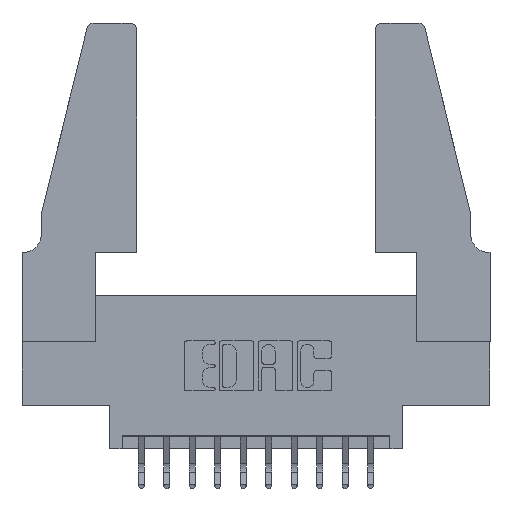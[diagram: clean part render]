
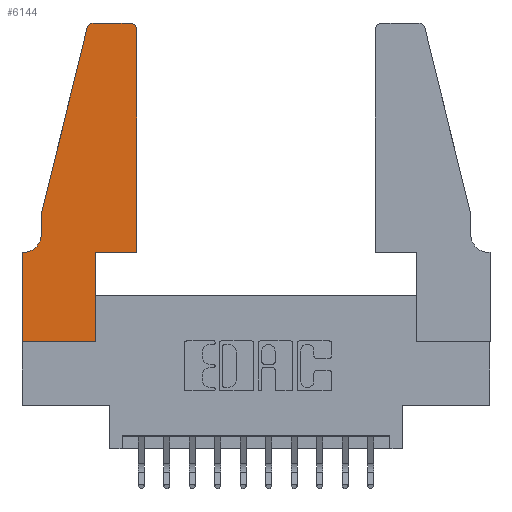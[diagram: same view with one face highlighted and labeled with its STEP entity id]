
A CAD part, top view. The second image highlights one B-rep face of the part: STEP entity #6144.
In plain terms, the highlighted planar face has unit normal (0, 0, 1).
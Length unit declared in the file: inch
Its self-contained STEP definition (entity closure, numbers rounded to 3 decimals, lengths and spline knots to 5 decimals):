
#168 = LINE ( 'NONE', #5309, #11917 ) ;
#169 = CARTESIAN_POINT ( 'NONE',  ( 0.0055, 0.35, 0.37 ) ) ;
#407 = EDGE_CURVE ( 'NONE', #7025, #11559, #3150, .T. ) ;
#533 = DIRECTION ( 'NONE',  ( 1., 0., 0. ) ) ;
#986 = CARTESIAN_POINT ( 'NONE',  ( 0.4505, 1.22, 0.37 ) ) ;
#995 = EDGE_LOOP ( 'NONE', ( #4113, #4151, #4274, #4350, #4409, #4457, #4525, #4723, #4753, #4770, #4849, #4875 ) ) ;
#1064 = DIRECTION ( 'NONE',  ( 0., 0., 1. ) ) ;
#1070 = CARTESIAN_POINT ( 'NONE',  ( 0.0755, 0.42, 0.37 ) ) ;
#1139 = CIRCLE ( 'NONE', #1979, 0.07 ) ;
#1775 = EDGE_CURVE ( 'NONE', #12695, #11120, #4900, .T. ) ;
#1860 = VECTOR ( 'NONE', #6840, 39.37008 ) ;
#1902 = CARTESIAN_POINT ( 'NONE',  ( 0.4205, 1.25, 0.37 ) ) ;
#1979 = AXIS2_PLACEMENT_3D ( 'NONE', #4079, #11868, #5188 ) ;
#2409 = EDGE_CURVE ( 'NONE', #10129, #10634, #13454, .T. ) ;
#2647 = EDGE_CURVE ( 'NONE', #4842, #14044, #4719, .T. ) ;
#3150 = LINE ( 'NONE', #5329, #8751 ) ;
#3224 = DIRECTION ( 'NONE',  ( 0., -1., 0. ) ) ;
#3579 = VERTEX_POINT ( 'NONE', #986 ) ;
#3812 = EDGE_CURVE ( 'NONE', #10634, #3579, #11188, .T. ) ;
#4055 = CARTESIAN_POINT ( 'NONE',  ( 0., 0.35, 0.37 ) ) ;
#4079 = CARTESIAN_POINT ( 'NONE',  ( 0.0055, 0.42, 0.37 ) ) ;
#4113 = ORIENTED_EDGE ( 'NONE', *, *, #12230, .T. ) ;
#4151 = ORIENTED_EDGE ( 'NONE', *, *, #2647, .T. ) ;
#4274 = ORIENTED_EDGE ( 'NONE', *, *, #13954, .T. ) ;
#4350 = ORIENTED_EDGE ( 'NONE', *, *, #1775, .T. ) ;
#4362 = VECTOR ( 'NONE', #4986, 39.37008 ) ;
#4409 = ORIENTED_EDGE ( 'NONE', *, *, #9693, .T. ) ;
#4457 = ORIENTED_EDGE ( 'NONE', *, *, #407, .T. ) ;
#4491 = VERTEX_POINT ( 'NONE', #4540 ) ;
#4525 = ORIENTED_EDGE ( 'NONE', *, *, #8069, .T. ) ;
#4540 = CARTESIAN_POINT ( 'NONE',  ( 0.2865, 0., 0.37 ) ) ;
#4719 = CIRCLE ( 'NONE', #12074, 0.03 ) ;
#4723 = ORIENTED_EDGE ( 'NONE', *, *, #12781, .T. ) ;
#4753 = ORIENTED_EDGE ( 'NONE', *, *, #14152, .T. ) ;
#4770 = ORIENTED_EDGE ( 'NONE', *, *, #2409, .T. ) ;
#4842 = VERTEX_POINT ( 'NONE', #10704 ) ;
#4849 = ORIENTED_EDGE ( 'NONE', *, *, #3812, .T. ) ;
#4875 = ORIENTED_EDGE ( 'NONE', *, *, #8145, .T. ) ;
#4900 = LINE ( 'NONE', #14087, #13107 ) ;
#4986 = DIRECTION ( 'NONE',  ( -0.239, -0.971, 0. ) ) ;
#5111 = PLANE ( 'NONE',  #6450 ) ;
#5149 = CARTESIAN_POINT ( 'NONE',  ( 0., 0., 0.37 ) ) ;
#5188 = DIRECTION ( 'NONE',  ( -1., 0., 0. ) ) ;
#5261 = LINE ( 'NONE', #5149, #10844 ) ;
#5309 = CARTESIAN_POINT ( 'NONE',  ( 0.2605, 1.25, 0.37 ) ) ;
#5329 = CARTESIAN_POINT ( 'NONE',  ( 0.0755, 0.35, 0.37 ) ) ;
#5587 = VERTEX_POINT ( 'NONE', #1902 ) ;
#5948 = CARTESIAN_POINT ( 'NONE',  ( 0.2865, 0.35, 0.37 ) ) ;
#6144 = ADVANCED_FACE ( 'NONE', ( #10615 ), #5111, .T. ) ;
#6252 = DIRECTION ( 'NONE',  ( 1., 0., 0. ) ) ;
#6427 = DIRECTION ( 'NONE',  ( -1., 0., 0. ) ) ;
#6450 = AXIS2_PLACEMENT_3D ( 'NONE', #4055, #7343, #533 ) ;
#6479 = AXIS2_PLACEMENT_3D ( 'NONE', #7821, #1064, #8996 ) ;
#6564 = CARTESIAN_POINT ( 'NONE',  ( 0., 0., 0.37 ) ) ;
#6840 = DIRECTION ( 'NONE',  ( 1., 0., 0. ) ) ;
#6867 = CARTESIAN_POINT ( 'NONE',  ( 0.4505, 0.35, 0.37 ) ) ;
#7025 = VERTEX_POINT ( 'NONE', #169 ) ;
#7343 = DIRECTION ( 'NONE',  ( 0., 0., 1. ) ) ;
#7460 = DIRECTION ( 'NONE',  ( 0., 1., 0. ) ) ;
#7719 = LINE ( 'NONE', #6564, #10383 ) ;
#7821 = CARTESIAN_POINT ( 'NONE',  ( 0.4205, 1.22, 0.37 ) ) ;
#8069 = EDGE_CURVE ( 'NONE', #11559, #12562, #7719, .T. ) ;
#8137 = VECTOR ( 'NONE', #13088, 39.37008 ) ;
#8145 = EDGE_CURVE ( 'NONE', #3579, #5587, #12330, .T. ) ;
#8181 = VECTOR ( 'NONE', #7460, 39.37008 ) ;
#8602 = CARTESIAN_POINT ( 'NONE',  ( 0.2865, 0.35, 0.37 ) ) ;
#8751 = VECTOR ( 'NONE', #6427, 39.37008 ) ;
#8996 = DIRECTION ( 'NONE',  ( 1., 0., 0. ) ) ;
#9260 = CARTESIAN_POINT ( 'NONE',  ( 0.4505, 0.35, 0.37 ) ) ;
#9693 = EDGE_CURVE ( 'NONE', #11120, #7025, #1139, .T. ) ;
#10129 = VERTEX_POINT ( 'NONE', #5948 ) ;
#10277 = CARTESIAN_POINT ( 'NONE',  ( 0., 0., 0.37 ) ) ;
#10383 = VECTOR ( 'NONE', #3224, 39.37008 ) ;
#10529 = CARTESIAN_POINT ( 'NONE',  ( 0.0755, 0.5, 0.37 ) ) ;
#10615 = FACE_OUTER_BOUND ( 'NONE', #995, .T. ) ;
#10634 = VERTEX_POINT ( 'NONE', #9260 ) ;
#10704 = CARTESIAN_POINT ( 'NONE',  ( 0.284, 1.25, 0.37 ) ) ;
#10840 = CARTESIAN_POINT ( 'NONE',  ( 0., 0.35, 0.37 ) ) ;
#10844 = VECTOR ( 'NONE', #6252, 39.37008 ) ;
#11120 = VERTEX_POINT ( 'NONE', #1070 ) ;
#11151 = DIRECTION ( 'NONE',  ( 0., -1., 0. ) ) ;
#11188 = LINE ( 'NONE', #13098, #8181 ) ;
#11559 = VERTEX_POINT ( 'NONE', #10840 ) ;
#11762 = CARTESIAN_POINT ( 'NONE',  ( 0.25487, 1.22718, 0.37 ) ) ;
#11868 = DIRECTION ( 'NONE',  ( 0., 0., -1. ) ) ;
#11917 = VECTOR ( 'NONE', #12011, 39.37008 ) ;
#12011 = DIRECTION ( 'NONE',  ( -1., 0., 0. ) ) ;
#12074 = AXIS2_PLACEMENT_3D ( 'NONE', #13768, #12428, #12373 ) ;
#12230 = EDGE_CURVE ( 'NONE', #5587, #4842, #168, .T. ) ;
#12330 = CIRCLE ( 'NONE', #6479, 0.03 ) ;
#12373 = DIRECTION ( 'NONE',  ( 1., 0., 0. ) ) ;
#12428 = DIRECTION ( 'NONE',  ( 0., 0., 1. ) ) ;
#12562 = VERTEX_POINT ( 'NONE', #10277 ) ;
#12695 = VERTEX_POINT ( 'NONE', #12780 ) ;
#12780 = CARTESIAN_POINT ( 'NONE',  ( 0.0755, 0.5, 0.37 ) ) ;
#12781 = EDGE_CURVE ( 'NONE', #12562, #4491, #5261, .T. ) ;
#13088 = DIRECTION ( 'NONE',  ( 0., 1., 0. ) ) ;
#13098 = CARTESIAN_POINT ( 'NONE',  ( 0.4505, 0.35, 0.37 ) ) ;
#13107 = VECTOR ( 'NONE', #11151, 39.37008 ) ;
#13454 = LINE ( 'NONE', #6867, #1860 ) ;
#13618 = LINE ( 'NONE', #10529, #4362 ) ;
#13768 = CARTESIAN_POINT ( 'NONE',  ( 0.284, 1.22, 0.37 ) ) ;
#13782 = LINE ( 'NONE', #8602, #8137 ) ;
#13954 = EDGE_CURVE ( 'NONE', #14044, #12695, #13618, .T. ) ;
#14044 = VERTEX_POINT ( 'NONE', #11762 ) ;
#14087 = CARTESIAN_POINT ( 'NONE',  ( 0.0755, 0.5, 0.37 ) ) ;
#14152 = EDGE_CURVE ( 'NONE', #4491, #10129, #13782, .T. ) ;
